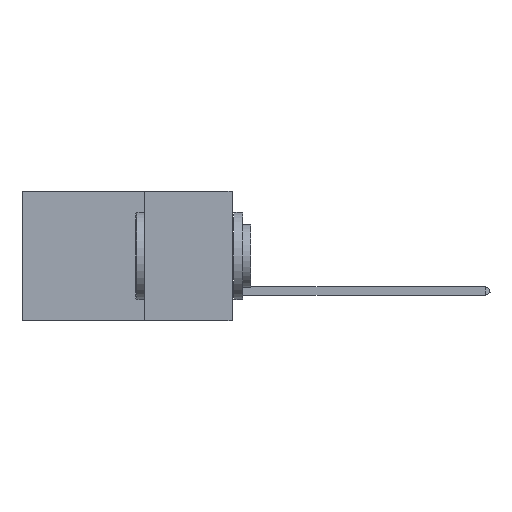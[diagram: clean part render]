
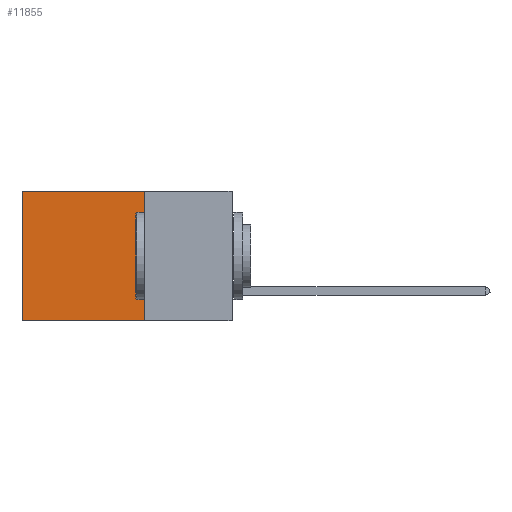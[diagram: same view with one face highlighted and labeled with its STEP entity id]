
A CAD part, left-side view. The second image highlights one B-rep face of the part: STEP entity #11855.
In plain terms, the highlighted planar face has unit normal (-1, 0, 0).
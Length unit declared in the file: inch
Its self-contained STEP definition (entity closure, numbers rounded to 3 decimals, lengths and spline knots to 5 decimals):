
#165 = CARTESIAN_POINT ( 'NONE',  ( 0.2875, 0.25, 0. ) ) ;
#1297 = CARTESIAN_POINT ( 'NONE',  ( 0.2875, 0.25, 0. ) ) ;
#2320 = FACE_OUTER_BOUND ( 'NONE', #13167, .T. ) ;
#3573 = VERTEX_POINT ( 'NONE', #165 ) ;
#4822 = CARTESIAN_POINT ( 'NONE',  ( 0.2875, 0.6, 0. ) ) ;
#5784 = PLANE ( 'NONE',  #17153 ) ;
#6366 = CARTESIAN_POINT ( 'NONE',  ( 0.2875, 0.25, 0. ) ) ;
#6545 = CARTESIAN_POINT ( 'NONE',  ( 0.2875, 0.25, -0.37 ) ) ;
#7466 = ORIENTED_EDGE ( 'NONE', *, *, #13691, .T. ) ;
#10087 = CARTESIAN_POINT ( 'NONE',  ( 0.2875, 0.25, -0.37 ) ) ;
#10110 = DIRECTION ( 'NONE',  ( 0., 0., -1. ) ) ;
#11380 = DIRECTION ( 'NONE',  ( 0., 1., 0. ) ) ;
#11855 = ADVANCED_FACE ( 'NONE', ( #2320 ), #5784, .F. ) ;
#12539 = DIRECTION ( 'NONE',  ( 1., 0., 0. ) ) ;
#13167 = EDGE_LOOP ( 'NONE', ( #7466, #29257, #20024, #24924 ) ) ;
#13691 = EDGE_CURVE ( 'NONE', #27767, #15528, #26930, .T. ) ;
#14011 = LINE ( 'NONE', #6545, #17240 ) ;
#14257 = VERTEX_POINT ( 'NONE', #10087 ) ;
#14307 = EDGE_CURVE ( 'NONE', #3573, #14257, #25080, .T. ) ;
#15102 = VECTOR ( 'NONE', #28778, 39.37008 ) ;
#15528 = VERTEX_POINT ( 'NONE', #27308 ) ;
#17153 = AXIS2_PLACEMENT_3D ( 'NONE', #19783, #12539, #10110 ) ;
#17240 = VECTOR ( 'NONE', #11380, 39.37008 ) ;
#18590 = VECTOR ( 'NONE', #20973, 39.37008 ) ;
#19758 = DIRECTION ( 'NONE',  ( 0., 0., -1. ) ) ;
#19783 = CARTESIAN_POINT ( 'NONE',  ( 0.2875, 0.25, 0. ) ) ;
#20024 = ORIENTED_EDGE ( 'NONE', *, *, #14307, .F. ) ;
#20476 = CARTESIAN_POINT ( 'NONE',  ( 0.2875, 0.6, 0. ) ) ;
#20973 = DIRECTION ( 'NONE',  ( 0., 0., -1. ) ) ;
#21223 = LINE ( 'NONE', #1297, #15102 ) ;
#21725 = EDGE_CURVE ( 'NONE', #14257, #15528, #14011, .T. ) ;
#24924 = ORIENTED_EDGE ( 'NONE', *, *, #26475, .T. ) ;
#25080 = LINE ( 'NONE', #6366, #25768 ) ;
#25768 = VECTOR ( 'NONE', #19758, 39.37008 ) ;
#26475 = EDGE_CURVE ( 'NONE', #3573, #27767, #21223, .T. ) ;
#26930 = LINE ( 'NONE', #4822, #18590 ) ;
#27308 = CARTESIAN_POINT ( 'NONE',  ( 0.2875, 0.6, -0.37 ) ) ;
#27767 = VERTEX_POINT ( 'NONE', #20476 ) ;
#28778 = DIRECTION ( 'NONE',  ( 0., 1., 0. ) ) ;
#29257 = ORIENTED_EDGE ( 'NONE', *, *, #21725, .F. ) ;
